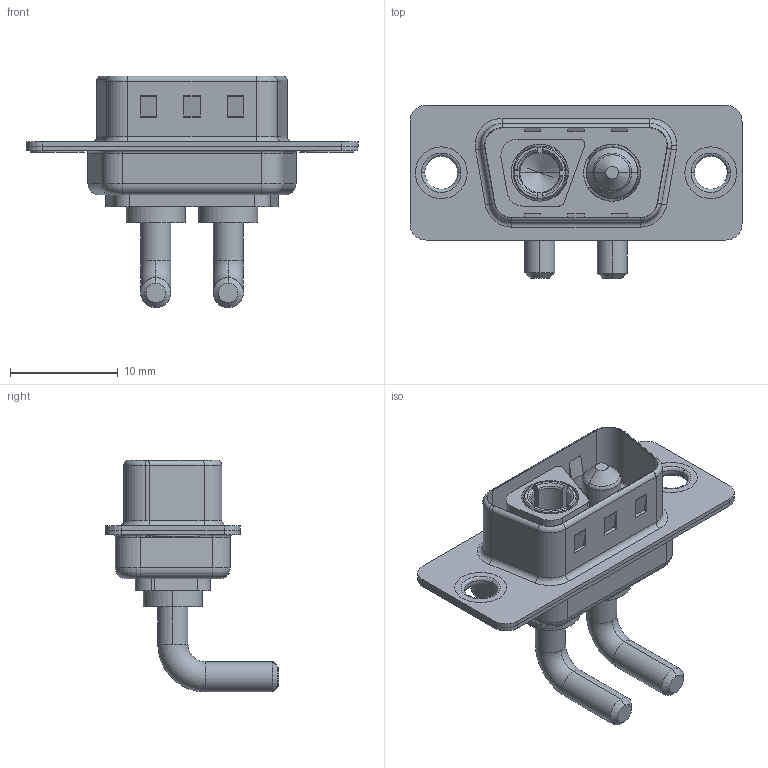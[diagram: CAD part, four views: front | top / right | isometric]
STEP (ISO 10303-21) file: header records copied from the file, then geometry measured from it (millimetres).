
FILE_DESCRIPTION (( 'STEP AP203' ), '1' );
FILE_NAME ('629-2WK2240-2N1.STEP', '2022-05-04T03:57:04', ( '' ), ( '' ), 'SwSTEP 2.0', 'SolidWorks 2020', '' );
FILE_SCHEMA (( 'CONFIG_CONTROL_DESIGN' ));
Length unit declared in the file: millimetre
Products named in the file (7): Power Socket_20A RA; 629Combo Thru Hole Rivet; Power Pin_20A RA; 629Combo Shell Rear_09 Contacts; 629Combo Housing_2WK2; 629-2WK2240-2N1; 629Combo Shell Front_09 Contacts
Assembly tree (7 placements, depth 2):
  629-2WK2240-2N1
    629Combo Housing_2WK2
    629Combo Shell Rear_09 Contacts
    629Combo Shell Front_09 Contacts
    629Combo Thru Hole Rivet  x2
    Power Socket_20A RA
    Power Pin_20A RA
Bounding box: 30.8 x 16.05 x 21.5 mm (x, y, z)
Volume: 1601.9 mm3; surface area: 3988 mm2
Topology: 9 solids, 9 shells, 409 faces, 1000 edges, 625 vertices
Faces by surface type: cylinder 164, plane 151, torus 68, cone 24, bspline 2
Entity records: 12544 total; most frequent: CARTESIAN_POINT 2288, DIRECTION 2124, ORIENTED_EDGE 1908, EDGE_CURVE 954, AXIS2_PLACEMENT_3D 828, VERTEX_POINT 601, VECTOR 468, LINE 468
